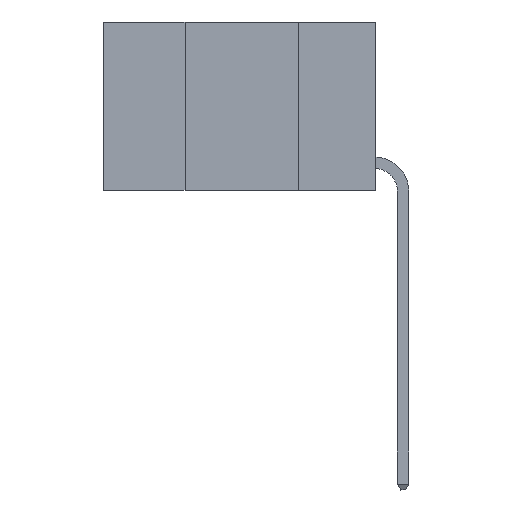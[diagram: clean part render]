
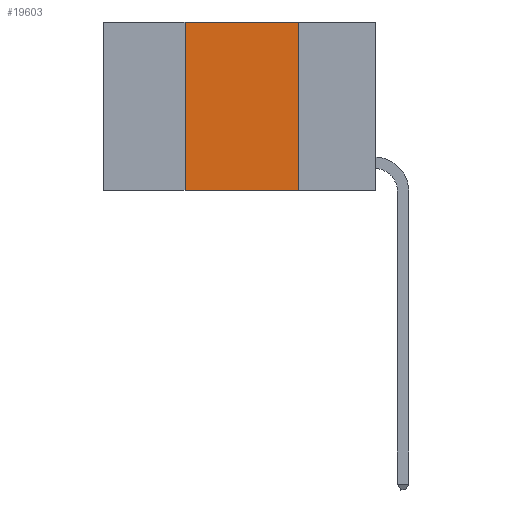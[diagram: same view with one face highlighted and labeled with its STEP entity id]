
A CAD part, left-side view. The second image highlights one B-rep face of the part: STEP entity #19603.
In plain terms, the highlighted planar face has unit normal (-1, 0, 0).
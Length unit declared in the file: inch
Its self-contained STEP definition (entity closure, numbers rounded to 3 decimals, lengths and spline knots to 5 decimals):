
#513 = LINE ( 'NONE', #2521, #31178 ) ;
#1049 = CARTESIAN_POINT ( 'NONE',  ( 0., 0.17, 0. ) ) ;
#1364 = DIRECTION ( 'NONE',  ( 1., 0., 0. ) ) ;
#1475 = DIRECTION ( 'NONE',  ( 0., -1., 0. ) ) ;
#1554 = ORIENTED_EDGE ( 'NONE', *, *, #27228, .F. ) ;
#2521 = CARTESIAN_POINT ( 'NONE',  ( 0., 0.17, 0. ) ) ;
#2785 = VERTEX_POINT ( 'NONE', #25179 ) ;
#3192 = EDGE_CURVE ( 'NONE', #15763, #15785, #513, .T. ) ;
#4282 = DIRECTION ( 'NONE',  ( 0., 0., 1. ) ) ;
#7317 = ORIENTED_EDGE ( 'NONE', *, *, #20349, .F. ) ;
#7456 = FACE_OUTER_BOUND ( 'NONE', #8477, .T. ) ;
#8477 = EDGE_LOOP ( 'NONE', ( #12963, #7317, #1554, #20922 ) ) ;
#9084 = CARTESIAN_POINT ( 'NONE',  ( 0., 0.42, 0. ) ) ;
#9299 = LINE ( 'NONE', #13587, #14959 ) ;
#10864 = VECTOR ( 'NONE', #11361, 39.37008 ) ;
#11361 = DIRECTION ( 'NONE',  ( 0., -1., 0. ) ) ;
#12963 = ORIENTED_EDGE ( 'NONE', *, *, #3192, .F. ) ;
#13587 = CARTESIAN_POINT ( 'NONE',  ( 0., 0.6, -0.37 ) ) ;
#13751 = CARTESIAN_POINT ( 'NONE',  ( 0., 0.6, 0. ) ) ;
#14156 = VERTEX_POINT ( 'NONE', #19425 ) ;
#14623 = DIRECTION ( 'NONE',  ( 0., 0., -1. ) ) ;
#14706 = VECTOR ( 'NONE', #4282, 39.37008 ) ;
#14959 = VECTOR ( 'NONE', #1475, 39.37008 ) ;
#15475 = LINE ( 'NONE', #9084, #14706 ) ;
#15763 = VERTEX_POINT ( 'NONE', #1049 ) ;
#15785 = VERTEX_POINT ( 'NONE', #18076 ) ;
#15930 = PLANE ( 'NONE',  #29063 ) ;
#18076 = CARTESIAN_POINT ( 'NONE',  ( 0., 0.17, -0.37 ) ) ;
#18387 = DIRECTION ( 'NONE',  ( 0., 0., -1. ) ) ;
#19425 = CARTESIAN_POINT ( 'NONE',  ( 0., 0.42, -0.37 ) ) ;
#19603 = ADVANCED_FACE ( 'NONE', ( #7456 ), #15930, .F. ) ;
#20349 = EDGE_CURVE ( 'NONE', #2785, #15763, #23664, .T. ) ;
#20922 = ORIENTED_EDGE ( 'NONE', *, *, #29155, .T. ) ;
#23664 = LINE ( 'NONE', #13751, #10864 ) ;
#25179 = CARTESIAN_POINT ( 'NONE',  ( 0., 0.42, 0. ) ) ;
#25489 = CARTESIAN_POINT ( 'NONE',  ( 0., 0.6, 0. ) ) ;
#27228 = EDGE_CURVE ( 'NONE', #14156, #2785, #15475, .T. ) ;
#29063 = AXIS2_PLACEMENT_3D ( 'NONE', #25489, #1364, #18387 ) ;
#29155 = EDGE_CURVE ( 'NONE', #14156, #15785, #9299, .T. ) ;
#31178 = VECTOR ( 'NONE', #14623, 39.37008 ) ;
